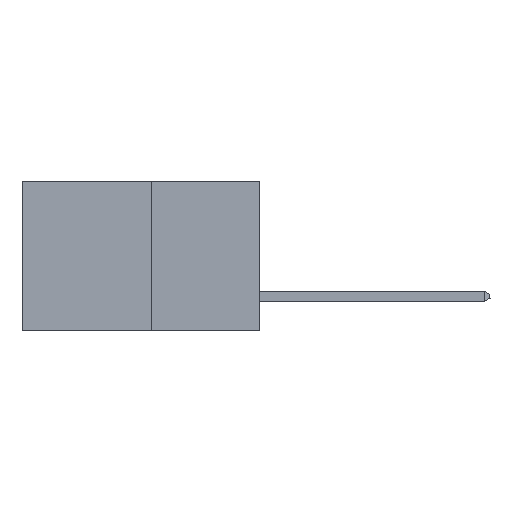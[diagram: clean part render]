
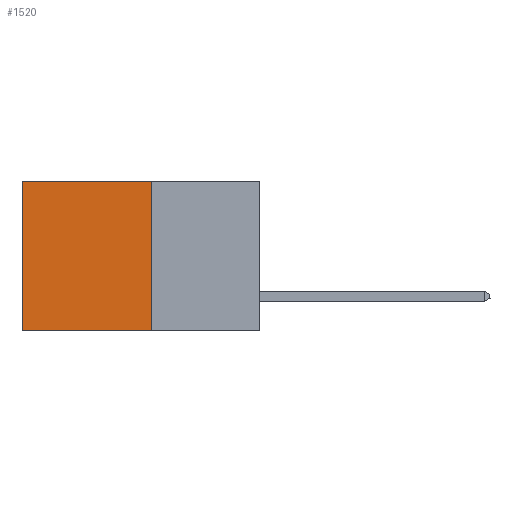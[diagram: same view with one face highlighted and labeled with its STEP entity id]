
A CAD part, left-side view. The second image highlights one B-rep face of the part: STEP entity #1520.
In plain terms, the highlighted planar face has unit normal (-1, 0, 0).
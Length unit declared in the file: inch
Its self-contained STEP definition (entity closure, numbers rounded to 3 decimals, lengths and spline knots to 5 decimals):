
#1237 = VECTOR ( 'NONE', #19501, 39.37008 ) ;
#1520 = ADVANCED_FACE ( 'NONE', ( #5894 ), #19663, .F. ) ;
#2107 = CARTESIAN_POINT ( 'NONE',  ( 0.277, 0.27, -0.37 ) ) ;
#2231 = EDGE_CURVE ( 'NONE', #7349, #30473, #3888, .T. ) ;
#3888 = LINE ( 'NONE', #30356, #29476 ) ;
#5640 = LINE ( 'NONE', #13099, #26217 ) ;
#5894 = FACE_OUTER_BOUND ( 'NONE', #22227, .T. ) ;
#7349 = VERTEX_POINT ( 'NONE', #16629 ) ;
#9514 = CARTESIAN_POINT ( 'NONE',  ( 0.277, 0.59, -0.37 ) ) ;
#9916 = EDGE_CURVE ( 'NONE', #7349, #15955, #5640, .T. ) ;
#10280 = ORIENTED_EDGE ( 'NONE', *, *, #2231, .F. ) ;
#11180 = ORIENTED_EDGE ( 'NONE', *, *, #22230, .F. ) ;
#11661 = DIRECTION ( 'NONE',  ( 1., 0., 0. ) ) ;
#11765 = ORIENTED_EDGE ( 'NONE', *, *, #9916, .T. ) ;
#11768 = DIRECTION ( 'NONE',  ( 0., 0., -1. ) ) ;
#12909 = CARTESIAN_POINT ( 'NONE',  ( 0.277, 0.59, 0. ) ) ;
#13099 = CARTESIAN_POINT ( 'NONE',  ( 0.277, 0.27, 0. ) ) ;
#13336 = CARTESIAN_POINT ( 'NONE',  ( 0.277, 0.59, -0.37 ) ) ;
#15450 = ORIENTED_EDGE ( 'NONE', *, *, #17836, .T. ) ;
#15955 = VERTEX_POINT ( 'NONE', #12909 ) ;
#16077 = VERTEX_POINT ( 'NONE', #13336 ) ;
#16629 = CARTESIAN_POINT ( 'NONE',  ( 0.277, 0.27, 0. ) ) ;
#16768 = VECTOR ( 'NONE', #27658, 39.37008 ) ;
#17836 = EDGE_CURVE ( 'NONE', #15955, #16077, #29178, .T. ) ;
#19501 = DIRECTION ( 'NONE',  ( 0., 0., -1. ) ) ;
#19574 = AXIS2_PLACEMENT_3D ( 'NONE', #2107, #11661, #11768 ) ;
#19663 = PLANE ( 'NONE',  #19574 ) ;
#22227 = EDGE_LOOP ( 'NONE', ( #15450, #11180, #10280, #11765 ) ) ;
#22230 = EDGE_CURVE ( 'NONE', #30473, #16077, #23340, .T. ) ;
#23340 = LINE ( 'NONE', #25112, #16768 ) ;
#25112 = CARTESIAN_POINT ( 'NONE',  ( 0.277, 0.27, -0.37 ) ) ;
#26195 = CARTESIAN_POINT ( 'NONE',  ( 0.277, 0.27, -0.37 ) ) ;
#26217 = VECTOR ( 'NONE', #30376, 39.37008 ) ;
#27658 = DIRECTION ( 'NONE',  ( 0., 1., 0. ) ) ;
#29178 = LINE ( 'NONE', #9514, #1237 ) ;
#29476 = VECTOR ( 'NONE', #29938, 39.37008 ) ;
#29938 = DIRECTION ( 'NONE',  ( 0., 0., -1. ) ) ;
#30356 = CARTESIAN_POINT ( 'NONE',  ( 0.277, 0.27, -0.37 ) ) ;
#30376 = DIRECTION ( 'NONE',  ( 0., 1., 0. ) ) ;
#30473 = VERTEX_POINT ( 'NONE', #26195 ) ;
